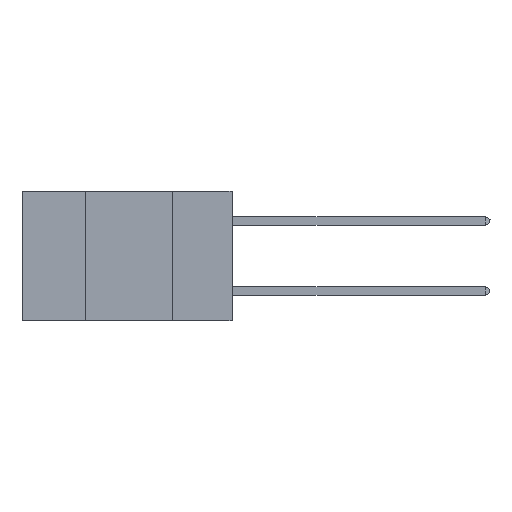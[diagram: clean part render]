
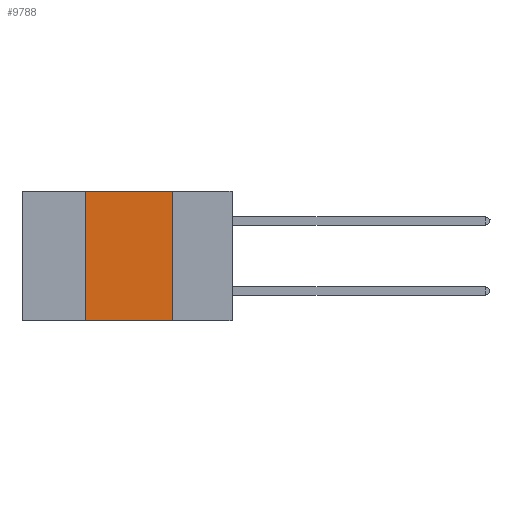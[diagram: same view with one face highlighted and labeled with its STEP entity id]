
A CAD part, left-side view. The second image highlights one B-rep face of the part: STEP entity #9788.
In plain terms, the highlighted planar face has unit normal (-1, 0, 0).
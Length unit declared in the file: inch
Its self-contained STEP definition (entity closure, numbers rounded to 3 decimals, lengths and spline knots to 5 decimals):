
#799 = DIRECTION ( 'NONE',  ( 0., -1., 0. ) ) ;
#1241 = VECTOR ( 'NONE', #799, 39.37008 ) ;
#1260 = CARTESIAN_POINT ( 'NONE',  ( 0., 0.42, 0. ) ) ;
#1370 = VERTEX_POINT ( 'NONE', #1260 ) ;
#1527 = LINE ( 'NONE', #6641, #9977 ) ;
#1769 = CARTESIAN_POINT ( 'NONE',  ( 0., 0.17, 0. ) ) ;
#2375 = EDGE_LOOP ( 'NONE', ( #10790, #11076, #6495, #3870 ) ) ;
#3229 = EDGE_CURVE ( 'NONE', #5515, #1370, #1527, .T. ) ;
#3328 = LINE ( 'NONE', #7520, #6426 ) ;
#3870 = ORIENTED_EDGE ( 'NONE', *, *, #12803, .T. ) ;
#4307 = EDGE_CURVE ( 'NONE', #11753, #10736, #7136, .T. ) ;
#4489 = CARTESIAN_POINT ( 'NONE',  ( 0., 0.42, -0.37 ) ) ;
#4985 = DIRECTION ( 'NONE',  ( 1., 0., 0. ) ) ;
#5515 = VERTEX_POINT ( 'NONE', #4489 ) ;
#6069 = EDGE_CURVE ( 'NONE', #1370, #11753, #3328, .T. ) ;
#6426 = VECTOR ( 'NONE', #6635, 39.37008 ) ;
#6495 = ORIENTED_EDGE ( 'NONE', *, *, #3229, .F. ) ;
#6635 = DIRECTION ( 'NONE',  ( 0., -1., 0. ) ) ;
#6641 = CARTESIAN_POINT ( 'NONE',  ( 0., 0.42, 0. ) ) ;
#6864 = LINE ( 'NONE', #6984, #1241 ) ;
#6912 = DIRECTION ( 'NONE',  ( 0., 0., 1. ) ) ;
#6984 = CARTESIAN_POINT ( 'NONE',  ( 0., 0.6, -0.37 ) ) ;
#6994 = AXIS2_PLACEMENT_3D ( 'NONE', #8102, #4985, #13261 ) ;
#7136 = LINE ( 'NONE', #1769, #8510 ) ;
#7520 = CARTESIAN_POINT ( 'NONE',  ( 0., 0.6, 0. ) ) ;
#7987 = DIRECTION ( 'NONE',  ( 0., 0., -1. ) ) ;
#8102 = CARTESIAN_POINT ( 'NONE',  ( 0., 0.6, 0. ) ) ;
#8510 = VECTOR ( 'NONE', #7987, 39.37008 ) ;
#8690 = CARTESIAN_POINT ( 'NONE',  ( 0., 0.17, 0. ) ) ;
#8982 = FACE_OUTER_BOUND ( 'NONE', #2375, .T. ) ;
#9467 = CARTESIAN_POINT ( 'NONE',  ( 0., 0.17, -0.37 ) ) ;
#9788 = ADVANCED_FACE ( 'NONE', ( #8982 ), #13136, .F. ) ;
#9977 = VECTOR ( 'NONE', #6912, 39.37008 ) ;
#10736 = VERTEX_POINT ( 'NONE', #9467 ) ;
#10790 = ORIENTED_EDGE ( 'NONE', *, *, #4307, .F. ) ;
#11076 = ORIENTED_EDGE ( 'NONE', *, *, #6069, .F. ) ;
#11753 = VERTEX_POINT ( 'NONE', #8690 ) ;
#12803 = EDGE_CURVE ( 'NONE', #5515, #10736, #6864, .T. ) ;
#13136 = PLANE ( 'NONE',  #6994 ) ;
#13261 = DIRECTION ( 'NONE',  ( 0., 0., -1. ) ) ;
